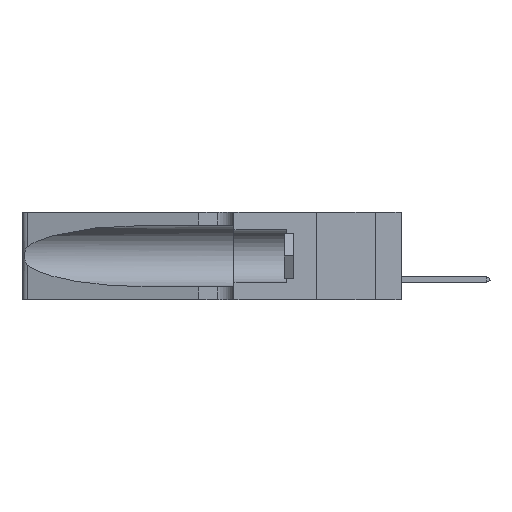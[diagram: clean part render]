
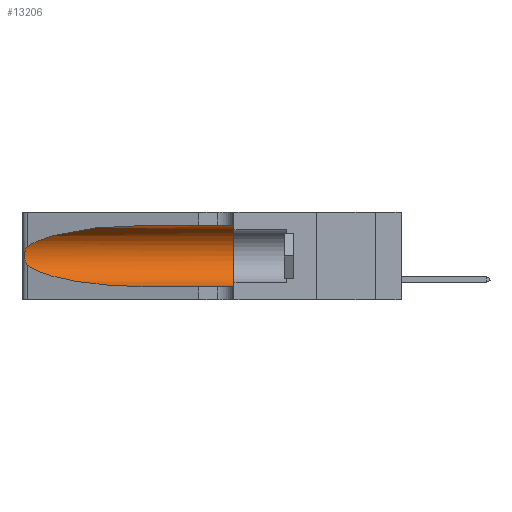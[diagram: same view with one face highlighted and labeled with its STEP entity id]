
A CAD part, left-side view. The second image highlights one B-rep face of the part: STEP entity #13206.
In plain terms, the highlighted cylindrical face has radius 3.308 mm (diameter 6.617 mm), a partial arc.
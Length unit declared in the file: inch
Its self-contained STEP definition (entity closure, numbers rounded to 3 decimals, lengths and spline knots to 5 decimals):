
#803 = EDGE_CURVE ( 'NONE', #3926, #17926, #26064, .T. ) ;
#906 = CYLINDRICAL_SURFACE ( 'NONE', #10402, 0.13025 ) ;
#910 = CARTESIAN_POINT ( 'NONE',  ( 0.1305, 1.61858, 0.185 ) ) ;
#2161 = CARTESIAN_POINT ( 'NONE',  ( 0.25487, 1.22718, 0.14631 ) ) ;
#2164 = VERTEX_POINT ( 'NONE', #24160 ) ;
#3206 = CARTESIAN_POINT ( 'NONE',  ( 0.26017, 1.23833, 0.17102 ) ) ;
#3485 = CARTESIAN_POINT ( 'NONE',  ( 0.1305, 0.72297, 0.31525 ) ) ;
#3552 = CARTESIAN_POINT ( 'NONE',  ( 0.1305, 1.61858, 0.05475 ) ) ;
#3926 = VERTEX_POINT ( 'NONE', #26479 ) ;
#5619 = FACE_OUTER_BOUND ( 'NONE', #28721, .T. ) ;
#6557 = DIRECTION ( 'NONE',  ( 0., -1., 0. ) ) ;
#6744 = CARTESIAN_POINT ( 'NONE',  ( 0.25487, 1.22718, 0.22369 ) ) ;
#6776 = CARTESIAN_POINT ( 'NONE',  ( 0.25854, 1.2359, 0.20912 ) ) ;
#6925 = CARTESIAN_POINT ( 'NONE',  ( 0.25555, 1.22994, 0.2215 ) ) ;
#8409 = DIRECTION ( 'NONE',  ( 0., -1., 0. ) ) ;
#9710 = EDGE_CURVE ( 'NONE', #27542, #2164, #12415, .T. ) ;
#10355 = CARTESIAN_POINT ( 'NONE',  ( 0.25787, 1.23484, 0.2124 ) ) ;
#10402 = AXIS2_PLACEMENT_3D ( 'NONE', #910, #8409, #46267 ) ;
#10900 = ORIENTED_EDGE ( 'NONE', *, *, #20183, .T. ) ;
#11156 = CIRCLE ( 'NONE', #14801, 0.13025 ) ;
#12415 = LINE ( 'NONE', #25288, #14781 ) ;
#12717 = B_SPLINE_CURVE_WITH_KNOTS ( 'NONE', 3,
 ( #33268, #6925, #32768, #10355, #6776, #40582, #14253, #17350, #3206, #21353, #25683, #47780, #14416, #25181 ),
 .UNSPECIFIED., .F., .F.,
 ( 4, 2, 2, 2, 2, 2, 4 ),
 ( 0., 0.00027, 0.00053, 0.00107, 0.0016, 0.00187, 0.00214 ),
 .UNSPECIFIED. ) ;
#12884 = CARTESIAN_POINT ( 'NONE',  ( 0.1305, 0.72297, 0.31525 ) ) ;
#13206 = ADVANCED_FACE ( 'NONE', ( #5619 ), #906, .F. ) ;
#13289 = CARTESIAN_POINT ( 'NONE',  ( 0.1305, 0.35, 0.185 ) ) ;
#14253 = CARTESIAN_POINT ( 'NONE',  ( 0.26075, 1.23896, 0.19203 ) ) ;
#14416 = CARTESIAN_POINT ( 'NONE',  ( 0.25555, 1.22993, 0.14849 ) ) ;
#14781 = VECTOR ( 'NONE', #6557, 39.37008 ) ;
#14801 = AXIS2_PLACEMENT_3D ( 'NONE', #13289, #39751, #17041 ) ;
#15118 = ORIENTED_EDGE ( 'NONE', *, *, #24963, .T. ) ;
#15965 = ORIENTED_EDGE ( 'NONE', *, *, #38300, .T. ) ;
#17041 = DIRECTION ( 'NONE',  ( 0., 0., 1. ) ) ;
#17350 = CARTESIAN_POINT ( 'NONE',  ( 0.26075, 1.23896, 0.178 ) ) ;
#17926 = VERTEX_POINT ( 'NONE', #48395 ) ;
#20183 = EDGE_CURVE ( 'NONE', #35813, #3926, #12717, .T. ) ;
#21110 = CARTESIAN_POINT ( 'NONE',  ( 0.18966, 0.96281, 0.05475 ) ) ;
#21353 = CARTESIAN_POINT ( 'NONE',  ( 0.25856, 1.23593, 0.16098 ) ) ;
#21367 = ORIENTED_EDGE ( 'NONE', *, *, #803, .T. ) ;
#21812 = CARTESIAN_POINT ( 'NONE',  ( 0.18966, 0.96281, 0.31525 ) ) ;
#22025 = ORIENTED_EDGE ( 'NONE', *, *, #26622, .F. ) ;
#24160 = CARTESIAN_POINT ( 'NONE',  ( 0.1305, 0.35, 0.31525 ) ) ;
#24395 = CARTESIAN_POINT ( 'NONE',  ( 0.25487, 1.22718, 0.22369 ) ) ;
#24937 = CARTESIAN_POINT ( 'NONE',  ( 0.1305, 0.72297, 0.05475 ) ) ;
#24963 = EDGE_CURVE ( 'NONE', #17926, #33934, #28170, .T. ) ;
#25181 = CARTESIAN_POINT ( 'NONE',  ( 0.25487, 1.22718, 0.14631 ) ) ;
#25288 = CARTESIAN_POINT ( 'NONE',  ( 0.1305, 1.61858, 0.31525 ) ) ;
#25683 = CARTESIAN_POINT ( 'NONE',  ( 0.25789, 1.23486, 0.15765 ) ) ;
#26064 =( BOUNDED_CURVE ( )  B_SPLINE_CURVE ( 3, ( #2161, #43613, #21110, #24937 ),
 .UNSPECIFIED., .F., .F. ) 
 B_SPLINE_CURVE_WITH_KNOTS ( ( 4, 4 ),
 ( 3.44316, 4.71239 ),
 .UNSPECIFIED. ) 
 CURVE ( )  GEOMETRIC_REPRESENTATION_ITEM ( )  RATIONAL_B_SPLINE_CURVE ( ( 1., 0.87, 0.87, 1. ) ) 
 REPRESENTATION_ITEM ( '' )  );
#26479 = CARTESIAN_POINT ( 'NONE',  ( 0.25487, 1.22718, 0.14631 ) ) ;
#26622 = EDGE_CURVE ( 'NONE', #2164, #33934, #11156, .T. ) ;
#27542 = VERTEX_POINT ( 'NONE', #12884 ) ;
#28170 = LINE ( 'NONE', #3552, #39424 ) ;
#28721 = EDGE_LOOP ( 'NONE', ( #15965, #10900, #21367, #15118, #22025, #47691 ) ) ;
#31182 =( BOUNDED_CURVE ( )  B_SPLINE_CURVE ( 3, ( #3485, #21812, #48586, #6744 ),
 .UNSPECIFIED., .F., .F. ) 
 B_SPLINE_CURVE_WITH_KNOTS ( ( 4, 4 ),
 ( 1.5708, 2.84003 ),
 .UNSPECIFIED. ) 
 CURVE ( )  GEOMETRIC_REPRESENTATION_ITEM ( )  RATIONAL_B_SPLINE_CURVE ( ( 1., 0.87, 0.87, 1. ) ) 
 REPRESENTATION_ITEM ( '' )  );
#32366 = CARTESIAN_POINT ( 'NONE',  ( 0.1305, 0.35, 0.05475 ) ) ;
#32768 = CARTESIAN_POINT ( 'NONE',  ( 0.25639, 1.23184, 0.21858 ) ) ;
#33268 = CARTESIAN_POINT ( 'NONE',  ( 0.25487, 1.22718, 0.22369 ) ) ;
#33934 = VERTEX_POINT ( 'NONE', #32366 ) ;
#35813 = VERTEX_POINT ( 'NONE', #24395 ) ;
#38300 = EDGE_CURVE ( 'NONE', #27542, #35813, #31182, .T. ) ;
#39424 = VECTOR ( 'NONE', #43602, 39.37008 ) ;
#39751 = DIRECTION ( 'NONE',  ( 0., 1., 0. ) ) ;
#40582 = CARTESIAN_POINT ( 'NONE',  ( 0.26018, 1.23835, 0.19895 ) ) ;
#43602 = DIRECTION ( 'NONE',  ( 0., -1., 0. ) ) ;
#43613 = CARTESIAN_POINT ( 'NONE',  ( 0.2373, 1.15595, 0.08982 ) ) ;
#46267 = DIRECTION ( 'NONE',  ( 0., 0., -1. ) ) ;
#47691 = ORIENTED_EDGE ( 'NONE', *, *, #9710, .F. ) ;
#47780 = CARTESIAN_POINT ( 'NONE',  ( 0.25639, 1.23186, 0.15144 ) ) ;
#48395 = CARTESIAN_POINT ( 'NONE',  ( 0.1305, 0.72297, 0.05475 ) ) ;
#48586 = CARTESIAN_POINT ( 'NONE',  ( 0.2373, 1.15595, 0.28018 ) ) ;
